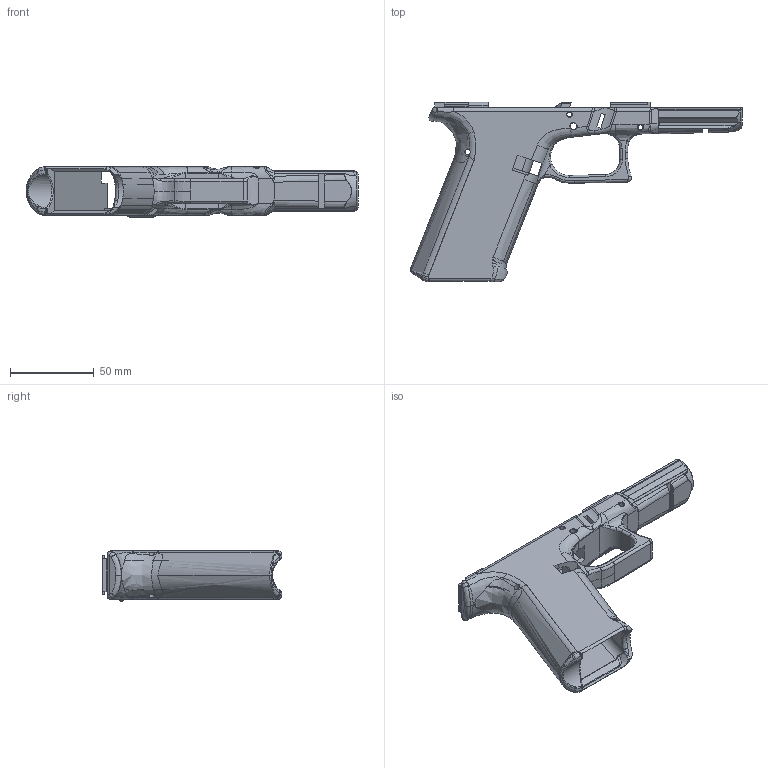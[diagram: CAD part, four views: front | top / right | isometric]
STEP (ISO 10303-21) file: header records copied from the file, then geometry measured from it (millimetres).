
FILE_DESCRIPTION(/* description */ (''),/* implementation_level */ '2;1');
FILE_NAME(/* name */ 'FMDA DD17.2 Assembly.stp',/* time_stamp */ '2021-01-10T11:55:08-06:00',/* author */ ('johne'),/* organization */ (''),/* preprocessor_version */ 'ST-DEVELOPER v18',/* originating_system */ 'Autodesk Inventor 2020',/* authorisation */ '');
FILE_SCHEMA (('AUTOMOTIVE_DESIGN { 1 0 10303 214 3 1 1 }'));
Products named in the file (4): FMDA DD17.2 Assembly; FMDA DD17.2 V1.4 Frame; Revised v2.0 rear rails - uniform profile - 45deg brace (2); FreeMans Glock 19
Assembly tree (3 placements, depth 2):
  FMDA DD17.2 Assembly
    FMDA DD17.2 V1.4 Frame
    Revised v2.0 rear rails - uniform profile - 45deg brace (2)
    FreeMans Glock 19
Bounding box: 197.63 x 106.75 x 29.84 mm (x, y, z)
Volume: 90975 mm3; surface area: 52464.7 mm2
Topology: 3 solids, 5 shells, 731 faces, 2045 edges, 1292 vertices
Faces by surface type: bspline 295, plane 228, cylinder 159, torus 21, sphere 16, cone 12
Full cylindrical faces by diameter (mm): 2 x1, 3 x5, 3.2 x4, 4 x2
Entity records: 53905 total; most frequent: CARTESIAN_POINT 36791, ORIENTED_EDGE 4066, DIRECTION 2898, EDGE_CURVE 2033, VERTEX_POINT 1293, AXIS2_PLACEMENT_3D 1039, LINE 820, VECTOR 820
